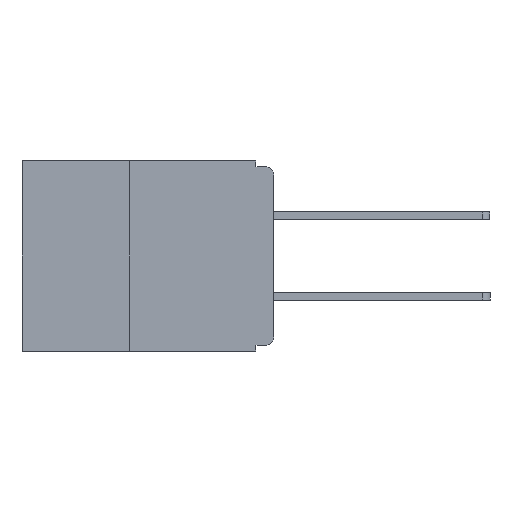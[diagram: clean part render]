
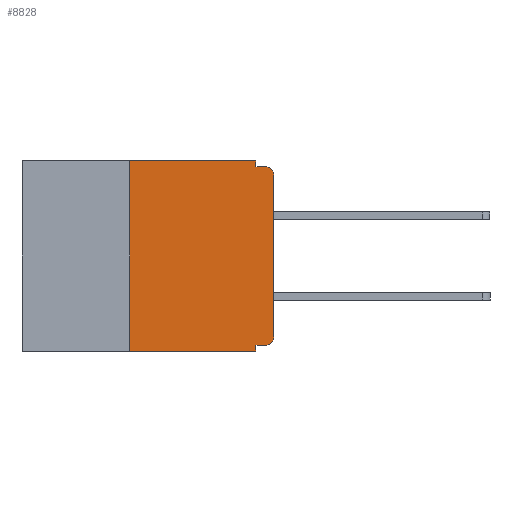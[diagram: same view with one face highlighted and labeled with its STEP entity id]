
A CAD part, left-side view. The second image highlights one B-rep face of the part: STEP entity #8828.
In plain terms, the highlighted planar face has unit normal (-1, 0, 0).
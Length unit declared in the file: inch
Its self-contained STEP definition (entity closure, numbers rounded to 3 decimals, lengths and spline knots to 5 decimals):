
#10 = PLANE ( 'NONE',  #5987 ) ;
#149 = ORIENTED_EDGE ( 'NONE', *, *, #5482, .T. ) ;
#727 = ORIENTED_EDGE ( 'NONE', *, *, #7857, .F. ) ;
#822 = LINE ( 'NONE', #20081, #14468 ) ;
#1178 = LINE ( 'NONE', #15148, #14255 ) ;
#1227 = AXIS2_PLACEMENT_3D ( 'NONE', #2885, #15285, #4670 ) ;
#1400 = DIRECTION ( 'NONE',  ( 0., 0., 1. ) ) ;
#1461 = VERTEX_POINT ( 'NONE', #2267 ) ;
#1484 = CARTESIAN_POINT ( 'NONE',  ( 0., 0., -0.32 ) ) ;
#1525 = CARTESIAN_POINT ( 'NONE',  ( 0., 0.25, -0.33 ) ) ;
#1886 = VECTOR ( 'NONE', #8298, 39.37008 ) ;
#1903 = EDGE_CURVE ( 'NONE', #1461, #9811, #14319, .T. ) ;
#2079 = VECTOR ( 'NONE', #3307, 39.37008 ) ;
#2267 = CARTESIAN_POINT ( 'NONE',  ( 0., 0.031, 0. ) ) ;
#2452 = LINE ( 'NONE', #4742, #1886 ) ;
#2753 = VERTEX_POINT ( 'NONE', #9886 ) ;
#2885 = CARTESIAN_POINT ( 'NONE',  ( 0., 0.015, -0.305 ) ) ;
#3129 = EDGE_CURVE ( 'NONE', #21113, #20476, #17016, .T. ) ;
#3307 = DIRECTION ( 'NONE',  ( 0., 1., 0. ) ) ;
#3548 = ORIENTED_EDGE ( 'NONE', *, *, #1903, .F. ) ;
#4250 = VERTEX_POINT ( 'NONE', #5684 ) ;
#4670 = DIRECTION ( 'NONE',  ( 0., 0., -1. ) ) ;
#4742 = CARTESIAN_POINT ( 'NONE',  ( 0., 0.437, 0. ) ) ;
#4975 = DIRECTION ( 'NONE',  ( -1., 0., 0. ) ) ;
#4993 = VERTEX_POINT ( 'NONE', #20543 ) ;
#5131 = VERTEX_POINT ( 'NONE', #15496 ) ;
#5388 = DIRECTION ( 'NONE',  ( 0., 0., -1. ) ) ;
#5472 = ORIENTED_EDGE ( 'NONE', *, *, #12879, .F. ) ;
#5482 = EDGE_CURVE ( 'NONE', #21113, #4993, #822, .T. ) ;
#5684 = CARTESIAN_POINT ( 'NONE',  ( 0., 0., -0.025 ) ) ;
#5987 = AXIS2_PLACEMENT_3D ( 'NONE', #17832, #7218, #19623 ) ;
#6787 = EDGE_CURVE ( 'NONE', #20476, #1461, #2452, .T. ) ;
#6826 = LINE ( 'NONE', #1484, #2079 ) ;
#7049 = VECTOR ( 'NONE', #1400, 39.37008 ) ;
#7218 = DIRECTION ( 'NONE',  ( 1., 0., 0. ) ) ;
#7702 = LINE ( 'NONE', #13005, #20751 ) ;
#7723 = CIRCLE ( 'NONE', #1227, 0.015 ) ;
#7729 = DIRECTION ( 'NONE',  ( 0., -1., 0. ) ) ;
#7857 = EDGE_CURVE ( 'NONE', #2753, #4993, #1178, .T. ) ;
#8298 = DIRECTION ( 'NONE',  ( 0., -1., 0. ) ) ;
#8367 = FACE_OUTER_BOUND ( 'NONE', #18665, .T. ) ;
#8807 = ORIENTED_EDGE ( 'NONE', *, *, #21188, .T. ) ;
#8828 = ADVANCED_FACE ( 'NONE', ( #8367 ), #10, .F. ) ;
#9753 = EDGE_CURVE ( 'NONE', #17048, #4250, #11119, .T. ) ;
#9811 = VERTEX_POINT ( 'NONE', #12285 ) ;
#9886 = CARTESIAN_POINT ( 'NONE',  ( 0., 0.031, -0.32 ) ) ;
#11119 = LINE ( 'NONE', #14109, #20030 ) ;
#11933 = ORIENTED_EDGE ( 'NONE', *, *, #9753, .T. ) ;
#12285 = CARTESIAN_POINT ( 'NONE',  ( 0., 0.031, -0.01 ) ) ;
#12879 = EDGE_CURVE ( 'NONE', #5131, #2753, #6826, .T. ) ;
#13005 = CARTESIAN_POINT ( 'NONE',  ( 0., 0., -0.01 ) ) ;
#13073 = CIRCLE ( 'NONE', #18724, 0.015 ) ;
#13410 = CARTESIAN_POINT ( 'NONE',  ( 0., 0.015, -0.01 ) ) ;
#13753 = ORIENTED_EDGE ( 'NONE', *, *, #6787, .F. ) ;
#14109 = CARTESIAN_POINT ( 'NONE',  ( 0., 0., 0. ) ) ;
#14255 = VECTOR ( 'NONE', #16933, 39.37008 ) ;
#14319 = LINE ( 'NONE', #22336, #18461 ) ;
#14468 = VECTOR ( 'NONE', #21785, 39.37008 ) ;
#14623 = ORIENTED_EDGE ( 'NONE', *, *, #3129, .F. ) ;
#15148 = CARTESIAN_POINT ( 'NONE',  ( 0., 0.031, -0.33 ) ) ;
#15174 = CARTESIAN_POINT ( 'NONE',  ( 0., 0.25, 0. ) ) ;
#15285 = DIRECTION ( 'NONE',  ( -1., 0., 0. ) ) ;
#15496 = CARTESIAN_POINT ( 'NONE',  ( 0., 0.015, -0.32 ) ) ;
#15573 = CARTESIAN_POINT ( 'NONE',  ( 0., 0., -0.305 ) ) ;
#15602 = CARTESIAN_POINT ( 'NONE',  ( 0., 0.015, -0.025 ) ) ;
#15875 = DIRECTION ( 'NONE',  ( 0., 0., 1. ) ) ;
#16455 = EDGE_CURVE ( 'NONE', #4250, #16898, #13073, .T. ) ;
#16898 = VERTEX_POINT ( 'NONE', #13410 ) ;
#16933 = DIRECTION ( 'NONE',  ( 0., 0., -1. ) ) ;
#17016 = LINE ( 'NONE', #1525, #7049 ) ;
#17048 = VERTEX_POINT ( 'NONE', #15573 ) ;
#17384 = DIRECTION ( 'NONE',  ( 0., 0., -1. ) ) ;
#17832 = CARTESIAN_POINT ( 'NONE',  ( 0., 0.437, 0. ) ) ;
#18461 = VECTOR ( 'NONE', #5388, 39.37008 ) ;
#18665 = EDGE_LOOP ( 'NONE', ( #11933, #21433, #20165, #3548, #13753, #14623, #149, #727, #5472, #8807 ) ) ;
#18724 = AXIS2_PLACEMENT_3D ( 'NONE', #15602, #4975, #17384 ) ;
#19623 = DIRECTION ( 'NONE',  ( 0., 0., -1. ) ) ;
#20030 = VECTOR ( 'NONE', #15875, 39.37008 ) ;
#20081 = CARTESIAN_POINT ( 'NONE',  ( 0., 0.437, -0.33 ) ) ;
#20165 = ORIENTED_EDGE ( 'NONE', *, *, #21610, .F. ) ;
#20476 = VERTEX_POINT ( 'NONE', #15174 ) ;
#20543 = CARTESIAN_POINT ( 'NONE',  ( 0., 0.031, -0.33 ) ) ;
#20751 = VECTOR ( 'NONE', #7729, 39.37008 ) ;
#21113 = VERTEX_POINT ( 'NONE', #21745 ) ;
#21188 = EDGE_CURVE ( 'NONE', #5131, #17048, #7723, .T. ) ;
#21433 = ORIENTED_EDGE ( 'NONE', *, *, #16455, .T. ) ;
#21610 = EDGE_CURVE ( 'NONE', #9811, #16898, #7702, .T. ) ;
#21745 = CARTESIAN_POINT ( 'NONE',  ( 0., 0.25, -0.33 ) ) ;
#21785 = DIRECTION ( 'NONE',  ( 0., -1., 0. ) ) ;
#22336 = CARTESIAN_POINT ( 'NONE',  ( 0., 0.031, 0. ) ) ;
